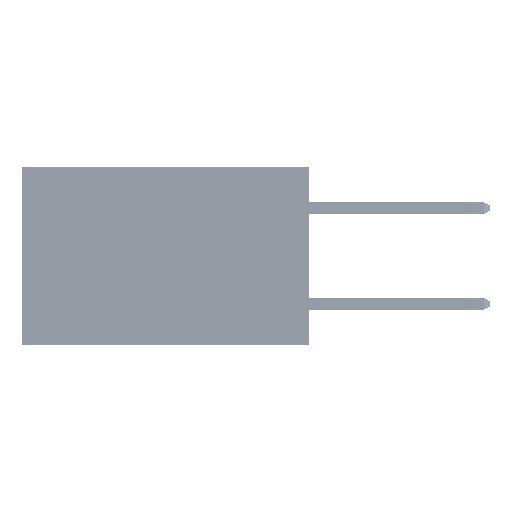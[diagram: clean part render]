
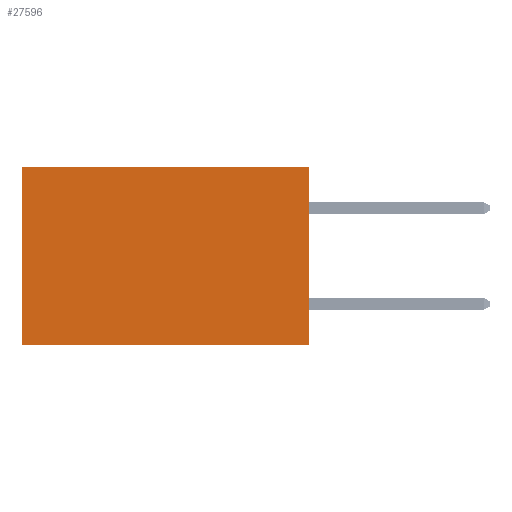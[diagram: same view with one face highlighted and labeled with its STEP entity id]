
A CAD part, left-side view. The second image highlights one B-rep face of the part: STEP entity #27596.
In plain terms, the highlighted planar face has unit normal (-1, 0, 0).
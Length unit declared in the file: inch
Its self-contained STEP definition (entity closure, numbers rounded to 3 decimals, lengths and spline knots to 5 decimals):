
#1444 = CARTESIAN_POINT ( 'NONE',  ( 0.2875, 0., 0. ) ) ;
#2879 = CARTESIAN_POINT ( 'NONE',  ( 0.2875, 0., -0.37 ) ) ;
#3133 = VERTEX_POINT ( 'NONE', #13268 ) ;
#6805 = VERTEX_POINT ( 'NONE', #1444 ) ;
#6886 = EDGE_CURVE ( 'NONE', #6805, #43441, #37810, .T. ) ;
#6913 = PLANE ( 'NONE',  #27345 ) ;
#8449 = EDGE_CURVE ( 'NONE', #31196, #3133, #32891, .T. ) ;
#8463 = VECTOR ( 'NONE', #32606, 39.37008 ) ;
#13268 = CARTESIAN_POINT ( 'NONE',  ( 0.2875, 0.6, -0.37 ) ) ;
#13682 = VECTOR ( 'NONE', #18905, 39.37008 ) ;
#14587 = CARTESIAN_POINT ( 'NONE',  ( 0.2875, 0., 0. ) ) ;
#18905 = DIRECTION ( 'NONE',  ( 0., 0., -1. ) ) ;
#19736 = CARTESIAN_POINT ( 'NONE',  ( 0.2875, 0.6, 0. ) ) ;
#21898 = DIRECTION ( 'NONE',  ( 0., 1., 0. ) ) ;
#24501 = EDGE_CURVE ( 'NONE', #43441, #3133, #30348, .T. ) ;
#25649 = DIRECTION ( 'NONE',  ( 0., 0., -1. ) ) ;
#26214 = EDGE_CURVE ( 'NONE', #6805, #31196, #29663, .T. ) ;
#27345 = AXIS2_PLACEMENT_3D ( 'NONE', #14587, #48616, #25649 ) ;
#27596 = ADVANCED_FACE ( 'NONE', ( #34899 ), #6913, .F. ) ;
#28605 = CARTESIAN_POINT ( 'NONE',  ( 0.2875, 0., -0.37 ) ) ;
#28767 = DIRECTION ( 'NONE',  ( 0., 1., 0. ) ) ;
#29663 = LINE ( 'NONE', #48879, #33832 ) ;
#30348 = LINE ( 'NONE', #28605, #49529 ) ;
#30583 = ORIENTED_EDGE ( 'NONE', *, *, #26214, .T. ) ;
#31196 = VERTEX_POINT ( 'NONE', #19736 ) ;
#32052 = ORIENTED_EDGE ( 'NONE', *, *, #24501, .F. ) ;
#32440 = CARTESIAN_POINT ( 'NONE',  ( 0.2875, 0., 0. ) ) ;
#32606 = DIRECTION ( 'NONE',  ( 0., 0., -1. ) ) ;
#32891 = LINE ( 'NONE', #33503, #13682 ) ;
#33503 = CARTESIAN_POINT ( 'NONE',  ( 0.2875, 0.6, 0. ) ) ;
#33832 = VECTOR ( 'NONE', #21898, 39.37008 ) ;
#34899 = FACE_OUTER_BOUND ( 'NONE', #47159, .T. ) ;
#37810 = LINE ( 'NONE', #32440, #8463 ) ;
#39387 = ORIENTED_EDGE ( 'NONE', *, *, #8449, .T. ) ;
#43441 = VERTEX_POINT ( 'NONE', #2879 ) ;
#47038 = ORIENTED_EDGE ( 'NONE', *, *, #6886, .F. ) ;
#47159 = EDGE_LOOP ( 'NONE', ( #39387, #32052, #47038, #30583 ) ) ;
#48616 = DIRECTION ( 'NONE',  ( 1., 0., 0. ) ) ;
#48879 = CARTESIAN_POINT ( 'NONE',  ( 0.2875, 0., 0. ) ) ;
#49529 = VECTOR ( 'NONE', #28767, 39.37008 ) ;
